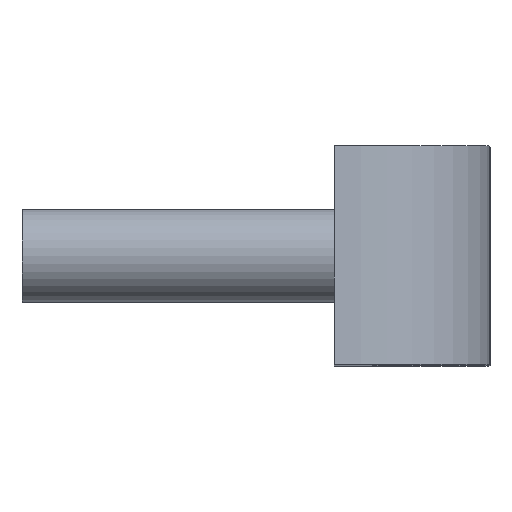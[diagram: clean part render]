
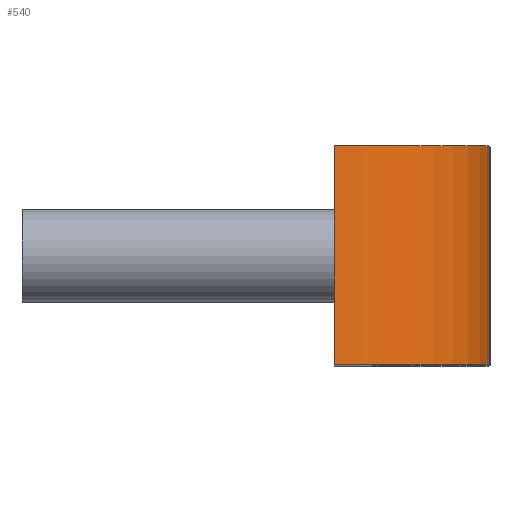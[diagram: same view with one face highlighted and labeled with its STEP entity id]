
A CAD part, top view. The second image highlights one B-rep face of the part: STEP entity #540.
In plain terms, the highlighted cylindrical face has radius 9.538 mm (diameter 19.075 mm), a partial arc.
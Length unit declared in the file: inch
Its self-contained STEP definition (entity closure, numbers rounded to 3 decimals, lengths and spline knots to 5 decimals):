
#5 = VERTEX_POINT ( 'NONE', #234 ) ;
#22 = EDGE_CURVE ( 'NONE', #97, #386, #609, .T. ) ;
#27 = CARTESIAN_POINT ( 'NONE',  ( -0.63193, 0.49, 0.96897 ) ) ;
#56 = VERTEX_POINT ( 'NONE', #312 ) ;
#73 = CARTESIAN_POINT ( 'NONE',  ( -0.3284, 0., 0.7479 ) ) ;
#86 = VECTOR ( 'NONE', #551, 39.37008 ) ;
#96 = CARTESIAN_POINT ( 'NONE',  ( -0.60632, 0.49, 1.34359 ) ) ;
#97 = VERTEX_POINT ( 'NONE', #73 ) ;
#103 = CARTESIAN_POINT ( 'NONE',  ( -0.3284, 0.49, 0.7479 ) ) ;
#111 = AXIS2_PLACEMENT_3D ( 'NONE', #176, #360, #534 ) ;
#139 = DIRECTION ( 'NONE',  ( 0., 1., 0. ) ) ;
#148 = AXIS2_PLACEMENT_3D ( 'NONE', #417, #504, #204 ) ;
#176 = CARTESIAN_POINT ( 'NONE',  ( -0.63193, 0.49, 0.96897 ) ) ;
#180 = VECTOR ( 'NONE', #338, 39.37008 ) ;
#196 = ORIENTED_EDGE ( 'NONE', *, *, #385, .F. ) ;
#204 = DIRECTION ( 'NONE',  ( 0., 0., 1. ) ) ;
#210 = CYLINDRICAL_SURFACE ( 'NONE', #111, 0.3755 ) ;
#217 = EDGE_LOOP ( 'NONE', ( #499, #413, #196, #333 ) ) ;
#234 = CARTESIAN_POINT ( 'NONE',  ( -0.60632, 0.49, 1.34359 ) ) ;
#241 = EDGE_CURVE ( 'NONE', #5, #56, #595, .T. ) ;
#312 = CARTESIAN_POINT ( 'NONE',  ( -0.60632, 0., 1.34359 ) ) ;
#315 = CARTESIAN_POINT ( 'NONE',  ( -0.3284, 0.49, 0.7479 ) ) ;
#333 = ORIENTED_EDGE ( 'NONE', *, *, #241, .T. ) ;
#338 = DIRECTION ( 'NONE',  ( 0., -1., 0. ) ) ;
#360 = DIRECTION ( 'NONE',  ( 0., -1., 0. ) ) ;
#385 = EDGE_CURVE ( 'NONE', #5, #386, #481, .T. ) ;
#386 = VERTEX_POINT ( 'NONE', #315 ) ;
#413 = ORIENTED_EDGE ( 'NONE', *, *, #22, .T. ) ;
#414 = FACE_OUTER_BOUND ( 'NONE', #217, .T. ) ;
#417 = CARTESIAN_POINT ( 'NONE',  ( -0.63193, 0., 0.96897 ) ) ;
#481 = CIRCLE ( 'NONE', #616, 0.3755 ) ;
#499 = ORIENTED_EDGE ( 'NONE', *, *, #544, .T. ) ;
#504 = DIRECTION ( 'NONE',  ( 0., 1., 0. ) ) ;
#534 = DIRECTION ( 'NONE',  ( 0., 0., -1. ) ) ;
#540 = ADVANCED_FACE ( 'NONE', ( #414 ), #210, .T. ) ;
#544 = EDGE_CURVE ( 'NONE', #56, #97, #568, .T. ) ;
#548 = DIRECTION ( 'NONE',  ( 0., 0., 1. ) ) ;
#551 = DIRECTION ( 'NONE',  ( 0., 1., 0. ) ) ;
#568 = CIRCLE ( 'NONE', #148, 0.3755 ) ;
#595 = LINE ( 'NONE', #96, #180 ) ;
#609 = LINE ( 'NONE', #103, #86 ) ;
#616 = AXIS2_PLACEMENT_3D ( 'NONE', #27, #139, #548 ) ;
